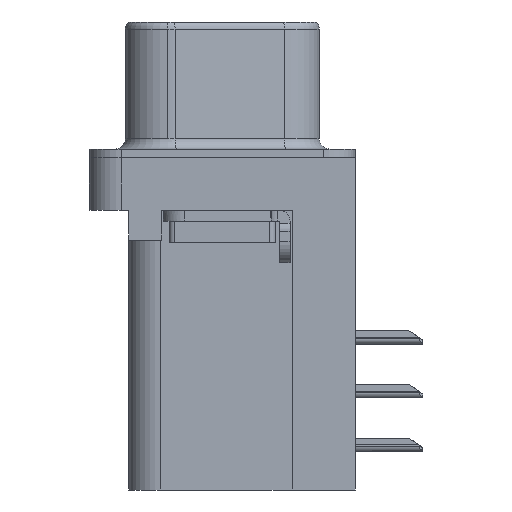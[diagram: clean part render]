
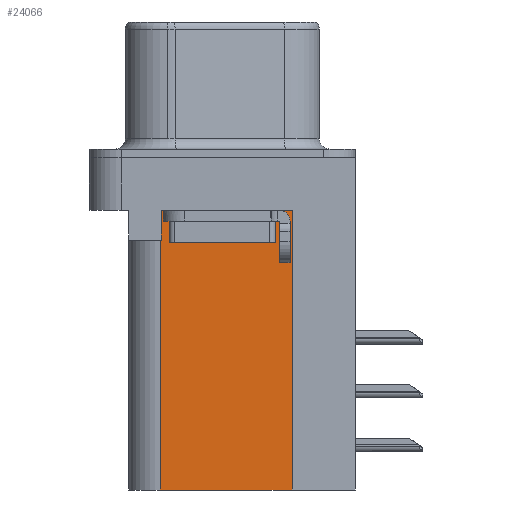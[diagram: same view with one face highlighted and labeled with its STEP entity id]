
A CAD part, left-side view. The second image highlights one B-rep face of the part: STEP entity #24066.
In plain terms, the highlighted planar face has unit normal (-1, 0, 0).
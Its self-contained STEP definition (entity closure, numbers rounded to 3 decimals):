
#3540 = LINE ( 'NONE', #7970, #31277 ) ;
#4792 = EDGE_CURVE ( 'NONE', #20521, #33652, #25780, .T. ) ;
#6296 = EDGE_CURVE ( 'NONE', #32123, #33652, #3540, .T. ) ;
#6518 = VECTOR ( 'NONE', #31258, 1000. ) ;
#6691 = LINE ( 'NONE', #9314, #34416 ) ;
#7066 = DIRECTION ( 'NONE',  ( 0., 1., 0. ) ) ;
#7437 = VERTEX_POINT ( 'NONE', #20249 ) ;
#7510 = CARTESIAN_POINT ( 'NONE',  ( 3.79, 0., -3.9 ) ) ;
#7593 = CARTESIAN_POINT ( 'NONE',  ( 3.79, -3.295, -2.5 ) ) ;
#7970 = CARTESIAN_POINT ( 'NONE',  ( 3.79, 2.925, -15.7 ) ) ;
#8362 = ORIENTED_EDGE ( 'NONE', *, *, #6296, .F. ) ;
#9185 = AXIS2_PLACEMENT_3D ( 'NONE', #21862, #11191, #27354 ) ;
#9314 = CARTESIAN_POINT ( 'NONE',  ( 3.79, -3.295, -15.7 ) ) ;
#10577 = CARTESIAN_POINT ( 'NONE',  ( 3.79, 2.925, -3.9 ) ) ;
#11191 = DIRECTION ( 'NONE',  ( 1., 0., 0. ) ) ;
#11821 = LINE ( 'NONE', #33133, #27754 ) ;
#12130 = EDGE_CURVE ( 'NONE', #17728, #20521, #20686, .T. ) ;
#13436 = CARTESIAN_POINT ( 'NONE',  ( 3.79, -3.295, -2.5 ) ) ;
#14380 = EDGE_CURVE ( 'NONE', #23405, #17728, #29461, .T. ) ;
#16175 = DIRECTION ( 'NONE',  ( 0., 0., 1. ) ) ;
#17084 = DIRECTION ( 'NONE',  ( 0., 1., 0. ) ) ;
#17728 = VERTEX_POINT ( 'NONE', #31858 ) ;
#18713 = VECTOR ( 'NONE', #7066, 1000. ) ;
#20249 = CARTESIAN_POINT ( 'NONE',  ( 3.79, -3.295, -15.7 ) ) ;
#20495 = ORIENTED_EDGE ( 'NONE', *, *, #20942, .F. ) ;
#20521 = VERTEX_POINT ( 'NONE', #31183 ) ;
#20686 = LINE ( 'NONE', #23194, #6518 ) ;
#20942 = EDGE_CURVE ( 'NONE', #7437, #32123, #11821, .T. ) ;
#21862 = CARTESIAN_POINT ( 'NONE',  ( 3.79, -3.295, -15.7 ) ) ;
#22213 = VECTOR ( 'NONE', #26855, 1000. ) ;
#23194 = CARTESIAN_POINT ( 'NONE',  ( 3.79, 2.895, -3.9 ) ) ;
#23405 = VERTEX_POINT ( 'NONE', #7593 ) ;
#23805 = CARTESIAN_POINT ( 'NONE',  ( 3.79, 2.925, -15.7 ) ) ;
#24066 = ADVANCED_FACE ( 'NONE', ( #30074 ), #24579, .F. ) ;
#24467 = EDGE_LOOP ( 'NONE', ( #30095, #26102, #34696, #8362, #20495, #34215 ) ) ;
#24579 = PLANE ( 'NONE',  #9185 ) ;
#25780 = LINE ( 'NONE', #7510, #18713 ) ;
#26102 = ORIENTED_EDGE ( 'NONE', *, *, #12130, .T. ) ;
#26855 = DIRECTION ( 'NONE',  ( 0., 1., 0. ) ) ;
#27354 = DIRECTION ( 'NONE',  ( 0., 0., -1. ) ) ;
#27754 = VECTOR ( 'NONE', #17084, 1000. ) ;
#28216 = EDGE_CURVE ( 'NONE', #7437, #23405, #6691, .T. ) ;
#29461 = LINE ( 'NONE', #13436, #22213 ) ;
#30074 = FACE_OUTER_BOUND ( 'NONE', #24467, .T. ) ;
#30095 = ORIENTED_EDGE ( 'NONE', *, *, #14380, .T. ) ;
#31183 = CARTESIAN_POINT ( 'NONE',  ( 3.79, 2.895, -3.9 ) ) ;
#31258 = DIRECTION ( 'NONE',  ( 0., 0., -1. ) ) ;
#31277 = VECTOR ( 'NONE', #16175, 1000. ) ;
#31858 = CARTESIAN_POINT ( 'NONE',  ( 3.79, 2.895, -2.5 ) ) ;
#32123 = VERTEX_POINT ( 'NONE', #23805 ) ;
#33133 = CARTESIAN_POINT ( 'NONE',  ( 3.79, -3.295, -15.7 ) ) ;
#33479 = DIRECTION ( 'NONE',  ( 0., 0., 1. ) ) ;
#33652 = VERTEX_POINT ( 'NONE', #10577 ) ;
#34215 = ORIENTED_EDGE ( 'NONE', *, *, #28216, .T. ) ;
#34416 = VECTOR ( 'NONE', #33479, 1000. ) ;
#34696 = ORIENTED_EDGE ( 'NONE', *, *, #4792, .T. ) ;
